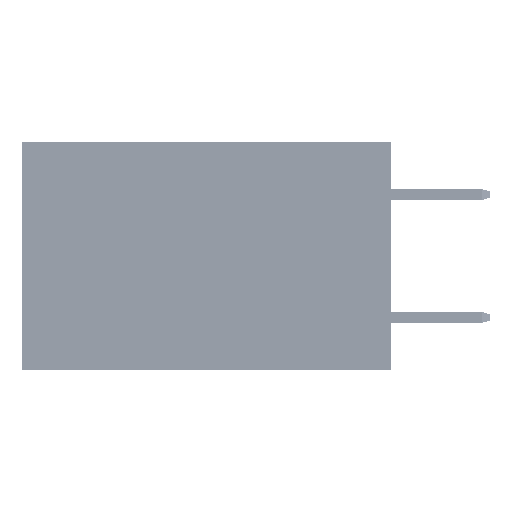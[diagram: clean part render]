
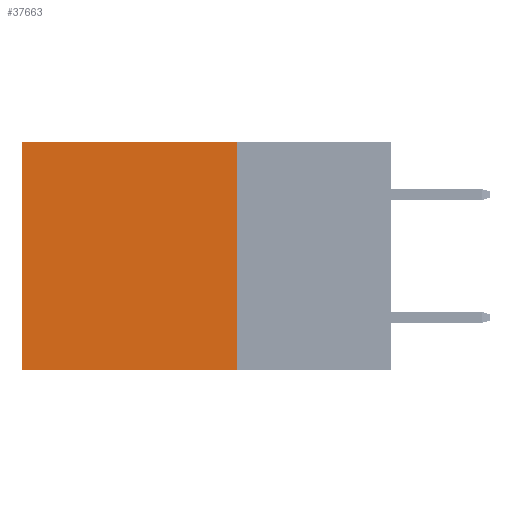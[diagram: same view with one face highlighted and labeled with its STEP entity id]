
A CAD part, left-side view. The second image highlights one B-rep face of the part: STEP entity #37663.
In plain terms, the highlighted planar face has unit normal (-1, 0, 0).
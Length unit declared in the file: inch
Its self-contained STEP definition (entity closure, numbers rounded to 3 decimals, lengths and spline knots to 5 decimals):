
#470 = PLANE ( 'NONE',  #35709 ) ;
#4633 = CARTESIAN_POINT ( 'NONE',  ( 0.2875, 0.25, 0. ) ) ;
#4750 = VERTEX_POINT ( 'NONE', #33365 ) ;
#5324 = EDGE_CURVE ( 'NONE', #11059, #4750, #9800, .T. ) ;
#7156 = CARTESIAN_POINT ( 'NONE',  ( 0.2875, 0.6, -0.37 ) ) ;
#7851 = CARTESIAN_POINT ( 'NONE',  ( 0.2875, 0.25, -0.37 ) ) ;
#8129 = EDGE_CURVE ( 'NONE', #11059, #41874, #10744, .T. ) ;
#9800 = LINE ( 'NONE', #16756, #52179 ) ;
#9912 = LINE ( 'NONE', #42977, #14972 ) ;
#10744 = LINE ( 'NONE', #4633, #20971 ) ;
#11059 = VERTEX_POINT ( 'NONE', #41914 ) ;
#12243 = DIRECTION ( 'NONE',  ( 0., 0., -1. ) ) ;
#14972 = VECTOR ( 'NONE', #22579, 39.37008 ) ;
#15039 = ORIENTED_EDGE ( 'NONE', *, *, #8129, .T. ) ;
#16027 = EDGE_CURVE ( 'NONE', #41874, #31379, #9912, .T. ) ;
#16336 = EDGE_CURVE ( 'NONE', #4750, #31379, #19453, .T. ) ;
#16756 = CARTESIAN_POINT ( 'NONE',  ( 0.2875, 0.25, 0. ) ) ;
#17133 = DIRECTION ( 'NONE',  ( 0., 1., 0. ) ) ;
#19453 = LINE ( 'NONE', #7851, #22014 ) ;
#20971 = VECTOR ( 'NONE', #17133, 39.37008 ) ;
#22014 = VECTOR ( 'NONE', #44491, 39.37008 ) ;
#22579 = DIRECTION ( 'NONE',  ( 0., 0., -1. ) ) ;
#23766 = CARTESIAN_POINT ( 'NONE',  ( 0.2875, 0.25, 0. ) ) ;
#29177 = ORIENTED_EDGE ( 'NONE', *, *, #16336, .F. ) ;
#31379 = VERTEX_POINT ( 'NONE', #7156 ) ;
#33365 = CARTESIAN_POINT ( 'NONE',  ( 0.2875, 0.25, -0.37 ) ) ;
#34098 = ORIENTED_EDGE ( 'NONE', *, *, #16027, .T. ) ;
#35709 = AXIS2_PLACEMENT_3D ( 'NONE', #23766, #49238, #12243 ) ;
#37663 = ADVANCED_FACE ( 'NONE', ( #45488 ), #470, .F. ) ;
#40219 = ORIENTED_EDGE ( 'NONE', *, *, #5324, .F. ) ;
#41874 = VERTEX_POINT ( 'NONE', #52528 ) ;
#41914 = CARTESIAN_POINT ( 'NONE',  ( 0.2875, 0.25, 0. ) ) ;
#42977 = CARTESIAN_POINT ( 'NONE',  ( 0.2875, 0.6, 0. ) ) ;
#44491 = DIRECTION ( 'NONE',  ( 0., 1., 0. ) ) ;
#45161 = EDGE_LOOP ( 'NONE', ( #34098, #29177, #40219, #15039 ) ) ;
#45488 = FACE_OUTER_BOUND ( 'NONE', #45161, .T. ) ;
#49238 = DIRECTION ( 'NONE',  ( 1., 0., 0. ) ) ;
#49633 = DIRECTION ( 'NONE',  ( 0., 0., -1. ) ) ;
#52179 = VECTOR ( 'NONE', #49633, 39.37008 ) ;
#52528 = CARTESIAN_POINT ( 'NONE',  ( 0.2875, 0.6, 0. ) ) ;
